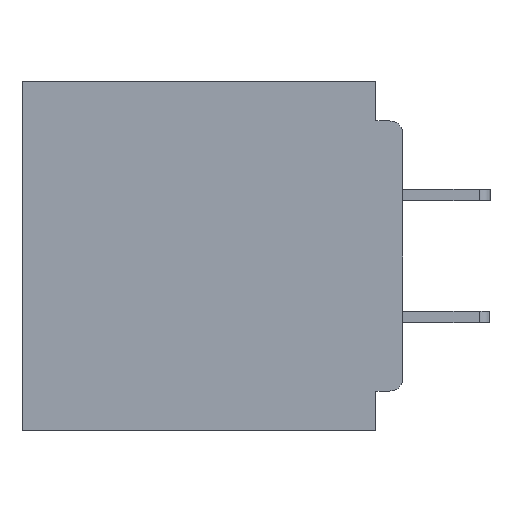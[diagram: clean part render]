
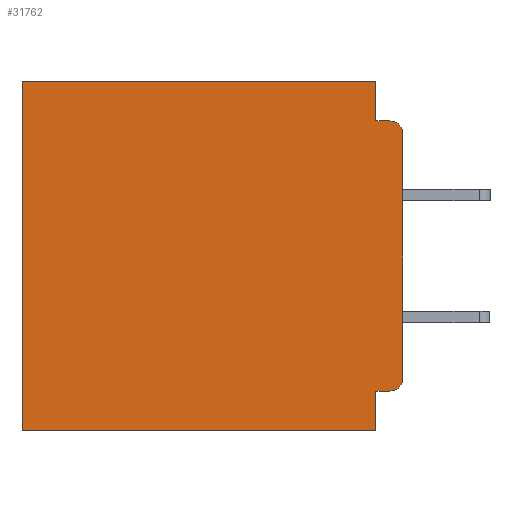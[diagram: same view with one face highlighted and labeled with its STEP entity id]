
A CAD part, left-side view. The second image highlights one B-rep face of the part: STEP entity #31762.
In plain terms, the highlighted planar face has unit normal (-1, 0, 0).
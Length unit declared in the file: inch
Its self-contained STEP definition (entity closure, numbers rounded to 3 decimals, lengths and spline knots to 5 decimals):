
#62 = DIRECTION ( 'NONE',  ( 1., 0., 0. ) ) ;
#646 = VECTOR ( 'NONE', #51629, 39.37008 ) ;
#2378 = VERTEX_POINT ( 'NONE', #42296 ) ;
#2390 = CARTESIAN_POINT ( 'NONE',  ( 0.3, 0.437, -0.4 ) ) ;
#3931 = EDGE_CURVE ( 'NONE', #48617, #5418, #10252, .T. ) ;
#5418 = VERTEX_POINT ( 'NONE', #34778 ) ;
#5985 = LINE ( 'NONE', #29470, #15101 ) ;
#6061 = VECTOR ( 'NONE', #56111, 39.37008 ) ;
#6556 = VERTEX_POINT ( 'NONE', #52414 ) ;
#6613 = FACE_OUTER_BOUND ( 'NONE', #46412, .T. ) ;
#6717 = CARTESIAN_POINT ( 'NONE',  ( 0.3, 0.031, 0. ) ) ;
#7565 = CARTESIAN_POINT ( 'NONE',  ( 0.3, 0., -0.4 ) ) ;
#8186 = EDGE_CURVE ( 'NONE', #13252, #26488, #24584, .T. ) ;
#8727 = ORIENTED_EDGE ( 'NONE', *, *, #8186, .F. ) ;
#8812 = DIRECTION ( 'NONE',  ( 0., 1., 0. ) ) ;
#9100 = CARTESIAN_POINT ( 'NONE',  ( 0.3, 0.015, -0.34 ) ) ;
#9205 = CIRCLE ( 'NONE', #38001, 0.015 ) ;
#9378 = CARTESIAN_POINT ( 'NONE',  ( 0.3, 0.015, -0.355 ) ) ;
#10252 = LINE ( 'NONE', #57215, #31374 ) ;
#10885 = DIRECTION ( 'NONE',  ( 0., 0., -1. ) ) ;
#12486 = ORIENTED_EDGE ( 'NONE', *, *, #15233, .F. ) ;
#13065 = CARTESIAN_POINT ( 'NONE',  ( 0.3, 0., -0.06 ) ) ;
#13252 = VERTEX_POINT ( 'NONE', #13065 ) ;
#13462 = CARTESIAN_POINT ( 'NONE',  ( 0.3, 0.015, -0.06 ) ) ;
#13567 = EDGE_CURVE ( 'NONE', #32634, #41483, #22466, .T. ) ;
#13577 = DIRECTION ( 'NONE',  ( 0., 0., -1. ) ) ;
#14804 = ORIENTED_EDGE ( 'NONE', *, *, #24485, .F. ) ;
#15101 = VECTOR ( 'NONE', #20423, 39.37008 ) ;
#15233 = EDGE_CURVE ( 'NONE', #5418, #18650, #26470, .T. ) ;
#15457 = EDGE_CURVE ( 'NONE', #47421, #26488, #50954, .T. ) ;
#16399 = DIRECTION ( 'NONE',  ( 0., 1., 0. ) ) ;
#16910 = ORIENTED_EDGE ( 'NONE', *, *, #38957, .F. ) ;
#18014 = DIRECTION ( 'NONE',  ( 0., 0., -1. ) ) ;
#18650 = VERTEX_POINT ( 'NONE', #28934 ) ;
#20292 = CARTESIAN_POINT ( 'NONE',  ( 0.3, 0., -0.4 ) ) ;
#20423 = DIRECTION ( 'NONE',  ( 0., -1., 0. ) ) ;
#22466 = LINE ( 'NONE', #37805, #33035 ) ;
#22490 = VECTOR ( 'NONE', #16399, 39.37008 ) ;
#22547 = VECTOR ( 'NONE', #8812, 39.37008 ) ;
#24485 = EDGE_CURVE ( 'NONE', #41483, #2378, #5985, .T. ) ;
#24584 = LINE ( 'NONE', #20292, #646 ) ;
#26470 = LINE ( 'NONE', #7565, #48873 ) ;
#26488 = VERTEX_POINT ( 'NONE', #39775 ) ;
#27006 = PLANE ( 'NONE',  #35538 ) ;
#28519 = CARTESIAN_POINT ( 'NONE',  ( 0.3, 0.031, -0.045 ) ) ;
#28934 = CARTESIAN_POINT ( 'NONE',  ( 0.3, 0.437, -0.4 ) ) ;
#29470 = CARTESIAN_POINT ( 'NONE',  ( 0.3, 0., -0.045 ) ) ;
#31374 = VECTOR ( 'NONE', #56803, 39.37008 ) ;
#31378 = ORIENTED_EDGE ( 'NONE', *, *, #15457, .T. ) ;
#31565 = DIRECTION ( 'NONE',  ( 0., 0., -1. ) ) ;
#31762 = ADVANCED_FACE ( 'NONE', ( #6613 ), #27006, .F. ) ;
#32624 = ORIENTED_EDGE ( 'NONE', *, *, #13567, .F. ) ;
#32634 = VERTEX_POINT ( 'NONE', #6717 ) ;
#33035 = VECTOR ( 'NONE', #10885, 39.37008 ) ;
#34356 = ORIENTED_EDGE ( 'NONE', *, *, #53776, .T. ) ;
#34475 = DIRECTION ( 'NONE',  ( 0., 1., 0. ) ) ;
#34519 = LINE ( 'NONE', #35709, #22547 ) ;
#34778 = CARTESIAN_POINT ( 'NONE',  ( 0.3, 0.031, -0.4 ) ) ;
#35538 = AXIS2_PLACEMENT_3D ( 'NONE', #44844, #62, #31565 ) ;
#35709 = CARTESIAN_POINT ( 'NONE',  ( 0.3, 0., 0. ) ) ;
#35768 = CARTESIAN_POINT ( 'NONE',  ( 0.3, 0.031, -0.355 ) ) ;
#37805 = CARTESIAN_POINT ( 'NONE',  ( 0.3, 0.031, 0. ) ) ;
#38001 = AXIS2_PLACEMENT_3D ( 'NONE', #13462, #44870, #18014 ) ;
#38513 = EDGE_CURVE ( 'NONE', #32634, #6556, #34519, .T. ) ;
#38535 = EDGE_CURVE ( 'NONE', #13252, #2378, #9205, .T. ) ;
#38957 = EDGE_CURVE ( 'NONE', #47421, #48617, #46313, .T. ) ;
#39050 = ORIENTED_EDGE ( 'NONE', *, *, #3931, .F. ) ;
#39775 = CARTESIAN_POINT ( 'NONE',  ( 0.3, 0., -0.34 ) ) ;
#40475 = DIRECTION ( 'NONE',  ( -1., 0., 0. ) ) ;
#41483 = VERTEX_POINT ( 'NONE', #28519 ) ;
#41854 = LINE ( 'NONE', #2390, #6061 ) ;
#42296 = CARTESIAN_POINT ( 'NONE',  ( 0.3, 0.015, -0.045 ) ) ;
#44844 = CARTESIAN_POINT ( 'NONE',  ( 0.3, 0., -0.4 ) ) ;
#44870 = DIRECTION ( 'NONE',  ( -1., 0., 0. ) ) ;
#45130 = ORIENTED_EDGE ( 'NONE', *, *, #38513, .T. ) ;
#45179 = ORIENTED_EDGE ( 'NONE', *, *, #38535, .T. ) ;
#46313 = LINE ( 'NONE', #56518, #22490 ) ;
#46412 = EDGE_LOOP ( 'NONE', ( #8727, #45179, #14804, #32624, #45130, #34356, #12486, #39050, #16910, #31378 ) ) ;
#47421 = VERTEX_POINT ( 'NONE', #9378 ) ;
#48617 = VERTEX_POINT ( 'NONE', #35768 ) ;
#48873 = VECTOR ( 'NONE', #34475, 39.37008 ) ;
#50954 = CIRCLE ( 'NONE', #53590, 0.015 ) ;
#51629 = DIRECTION ( 'NONE',  ( 0., 0., -1. ) ) ;
#52414 = CARTESIAN_POINT ( 'NONE',  ( 0.3, 0.437, 0. ) ) ;
#53590 = AXIS2_PLACEMENT_3D ( 'NONE', #9100, #40475, #13577 ) ;
#53776 = EDGE_CURVE ( 'NONE', #6556, #18650, #41854, .T. ) ;
#56111 = DIRECTION ( 'NONE',  ( 0., 0., -1. ) ) ;
#56518 = CARTESIAN_POINT ( 'NONE',  ( 0.3, 0., -0.355 ) ) ;
#56803 = DIRECTION ( 'NONE',  ( 0., 0., -1. ) ) ;
#57215 = CARTESIAN_POINT ( 'NONE',  ( 0.3, 0.031, -0.4 ) ) ;
